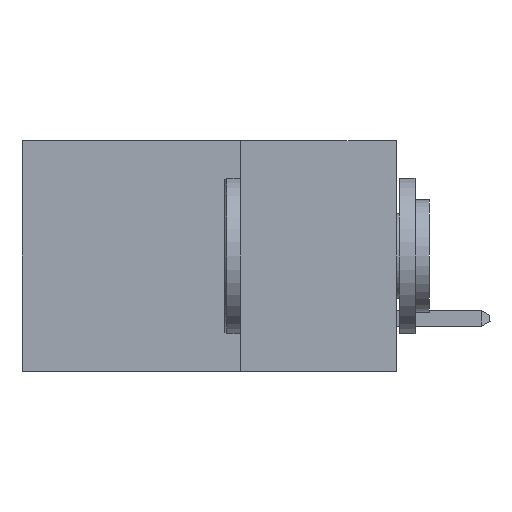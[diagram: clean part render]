
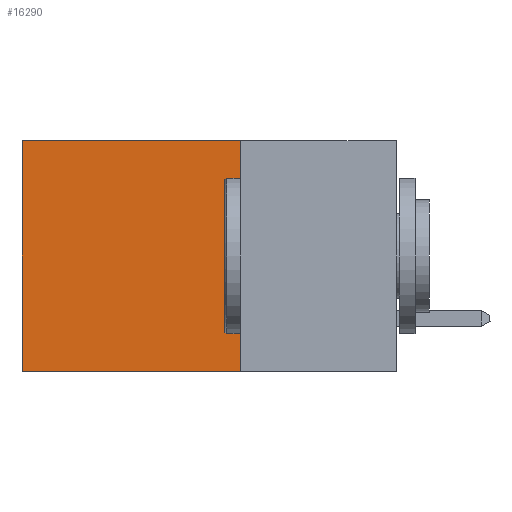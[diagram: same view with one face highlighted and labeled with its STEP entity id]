
A CAD part, left-side view. The second image highlights one B-rep face of the part: STEP entity #16290.
In plain terms, the highlighted planar face has unit normal (-1, 0, 0).
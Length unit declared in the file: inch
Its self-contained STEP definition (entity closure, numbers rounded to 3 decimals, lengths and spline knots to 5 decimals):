
#1885 = DIRECTION ( 'NONE',  ( 0., 0., -1. ) ) ;
#2910 = CARTESIAN_POINT ( 'NONE',  ( 0.298, 0.25, 0. ) ) ;
#2920 = EDGE_LOOP ( 'NONE', ( #3435, #19768, #23027, #19941 ) ) ;
#3435 = ORIENTED_EDGE ( 'NONE', *, *, #18453, .T. ) ;
#6916 = LINE ( 'NONE', #8772, #18493 ) ;
#7390 = AXIS2_PLACEMENT_3D ( 'NONE', #13448, #15256, #10216 ) ;
#7820 = VERTEX_POINT ( 'NONE', #19571 ) ;
#7987 = EDGE_CURVE ( 'NONE', #16047, #22230, #21472, .T. ) ;
#8045 = DIRECTION ( 'NONE',  ( 0., 1., 0. ) ) ;
#8439 = CARTESIAN_POINT ( 'NONE',  ( 0.298, 0.25, 0. ) ) ;
#8772 = CARTESIAN_POINT ( 'NONE',  ( 0.298, 0.6, 0. ) ) ;
#10030 = CARTESIAN_POINT ( 'NONE',  ( 0.298, 0.25, -0.37 ) ) ;
#10216 = DIRECTION ( 'NONE',  ( 0., 0., -1. ) ) ;
#11523 = VERTEX_POINT ( 'NONE', #10030 ) ;
#11641 = PLANE ( 'NONE',  #7390 ) ;
#11788 = CARTESIAN_POINT ( 'NONE',  ( 0.298, 0.25, -0.37 ) ) ;
#11909 = VECTOR ( 'NONE', #22953, 39.37008 ) ;
#13448 = CARTESIAN_POINT ( 'NONE',  ( 0.298, 0.25, 0. ) ) ;
#13814 = CARTESIAN_POINT ( 'NONE',  ( 0.298, 0.6, 0. ) ) ;
#14914 = FACE_OUTER_BOUND ( 'NONE', #2920, .T. ) ;
#15256 = DIRECTION ( 'NONE',  ( 1., 0., 0. ) ) ;
#15272 = VECTOR ( 'NONE', #22742, 39.37008 ) ;
#15785 = LINE ( 'NONE', #11788, #19982 ) ;
#15810 = CARTESIAN_POINT ( 'NONE',  ( 0.298, 0.25, 0. ) ) ;
#15910 = EDGE_CURVE ( 'NONE', #11523, #7820, #15785, .T. ) ;
#16047 = VERTEX_POINT ( 'NONE', #8439 ) ;
#16290 = ADVANCED_FACE ( 'NONE', ( #14914 ), #11641, .F. ) ;
#18453 = EDGE_CURVE ( 'NONE', #22230, #7820, #6916, .T. ) ;
#18493 = VECTOR ( 'NONE', #1885, 39.37008 ) ;
#18656 = LINE ( 'NONE', #2910, #15272 ) ;
#19571 = CARTESIAN_POINT ( 'NONE',  ( 0.298, 0.6, -0.37 ) ) ;
#19768 = ORIENTED_EDGE ( 'NONE', *, *, #15910, .F. ) ;
#19941 = ORIENTED_EDGE ( 'NONE', *, *, #7987, .T. ) ;
#19982 = VECTOR ( 'NONE', #8045, 39.37008 ) ;
#20829 = EDGE_CURVE ( 'NONE', #16047, #11523, #18656, .T. ) ;
#21472 = LINE ( 'NONE', #15810, #11909 ) ;
#22230 = VERTEX_POINT ( 'NONE', #13814 ) ;
#22742 = DIRECTION ( 'NONE',  ( 0., 0., -1. ) ) ;
#22953 = DIRECTION ( 'NONE',  ( 0., 1., 0. ) ) ;
#23027 = ORIENTED_EDGE ( 'NONE', *, *, #20829, .F. ) ;
